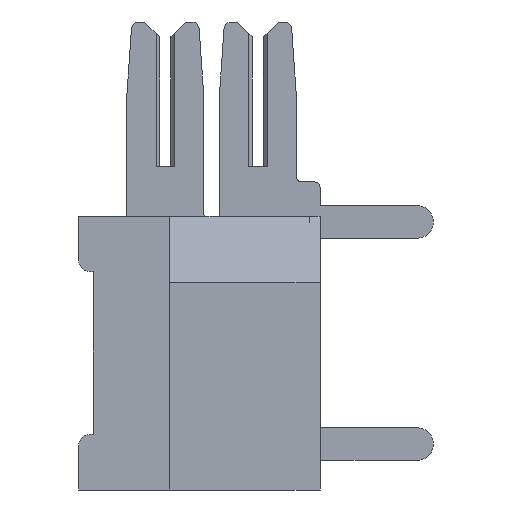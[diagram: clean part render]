
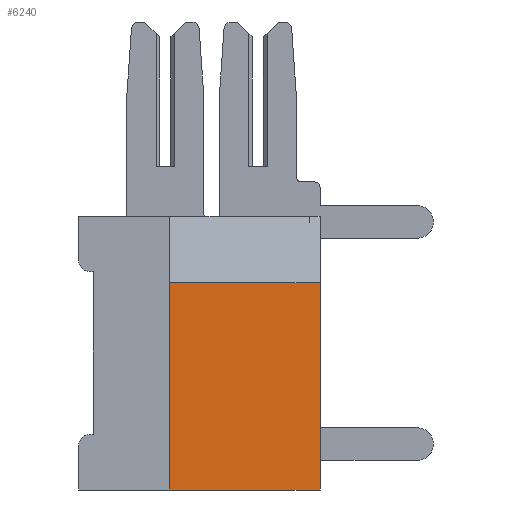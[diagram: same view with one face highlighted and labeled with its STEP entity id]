
A CAD part, left-side view. The second image highlights one B-rep face of the part: STEP entity #6240.
In plain terms, the highlighted planar face has unit normal (-1, 0, 0).
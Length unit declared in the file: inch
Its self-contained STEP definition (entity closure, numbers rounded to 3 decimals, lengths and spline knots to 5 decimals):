
#129 = LINE ( 'NONE', #5460, #4570 ) ;
#377 = LINE ( 'NONE', #6241, #7783 ) ;
#827 = CARTESIAN_POINT ( 'NONE',  ( 0., 0.326, -0.37 ) ) ;
#839 = ORIENTED_EDGE ( 'NONE', *, *, #5749, .T. ) ;
#1320 = EDGE_LOOP ( 'NONE', ( #839, #5356, #2176, #2453 ) ) ;
#1995 = VECTOR ( 'NONE', #5983, 39.37008 ) ;
#2176 = ORIENTED_EDGE ( 'NONE', *, *, #2248, .F. ) ;
#2248 = EDGE_CURVE ( 'NONE', #8248, #4870, #129, .T. ) ;
#2453 = ORIENTED_EDGE ( 'NONE', *, *, #7682, .T. ) ;
#2561 = AXIS2_PLACEMENT_3D ( 'NONE', #8354, #4419, #4464 ) ;
#2801 = FACE_OUTER_BOUND ( 'NONE', #1320, .T. ) ;
#3848 = PLANE ( 'NONE',  #2561 ) ;
#4419 = DIRECTION ( 'NONE',  ( 1., 0., 0. ) ) ;
#4464 = DIRECTION ( 'NONE',  ( 0., 0., -1. ) ) ;
#4557 = VERTEX_POINT ( 'NONE', #5108 ) ;
#4570 = VECTOR ( 'NONE', #7436, 39.37008 ) ;
#4797 = LINE ( 'NONE', #827, #7154 ) ;
#4870 = VERTEX_POINT ( 'NONE', #6760 ) ;
#5108 = CARTESIAN_POINT ( 'NONE',  ( 0., 0., -0.09 ) ) ;
#5342 = CARTESIAN_POINT ( 'NONE',  ( 0., 0., 0. ) ) ;
#5356 = ORIENTED_EDGE ( 'NONE', *, *, #6022, .T. ) ;
#5460 = CARTESIAN_POINT ( 'NONE',  ( 0., 0.203, -0.37 ) ) ;
#5548 = LINE ( 'NONE', #5342, #1995 ) ;
#5749 = EDGE_CURVE ( 'NONE', #5934, #4557, #5548, .T. ) ;
#5934 = VERTEX_POINT ( 'NONE', #7459 ) ;
#5983 = DIRECTION ( 'NONE',  ( 0., 0., 1. ) ) ;
#6022 = EDGE_CURVE ( 'NONE', #4557, #4870, #377, .T. ) ;
#6240 = ADVANCED_FACE ( 'NONE', ( #2801 ), #3848, .F. ) ;
#6241 = CARTESIAN_POINT ( 'NONE',  ( 0., 0., -0.09 ) ) ;
#6379 = CARTESIAN_POINT ( 'NONE',  ( 0., 0.203, -0.37 ) ) ;
#6760 = CARTESIAN_POINT ( 'NONE',  ( 0., 0.203, -0.09 ) ) ;
#7154 = VECTOR ( 'NONE', #7922, 39.37008 ) ;
#7436 = DIRECTION ( 'NONE',  ( 0., 0., 1. ) ) ;
#7459 = CARTESIAN_POINT ( 'NONE',  ( 0., 0., -0.37 ) ) ;
#7682 = EDGE_CURVE ( 'NONE', #8248, #5934, #4797, .T. ) ;
#7783 = VECTOR ( 'NONE', #8161, 39.37008 ) ;
#7922 = DIRECTION ( 'NONE',  ( 0., -1., 0. ) ) ;
#8161 = DIRECTION ( 'NONE',  ( 0., 1., 0. ) ) ;
#8248 = VERTEX_POINT ( 'NONE', #6379 ) ;
#8354 = CARTESIAN_POINT ( 'NONE',  ( 0., 0.326, 0. ) ) ;
